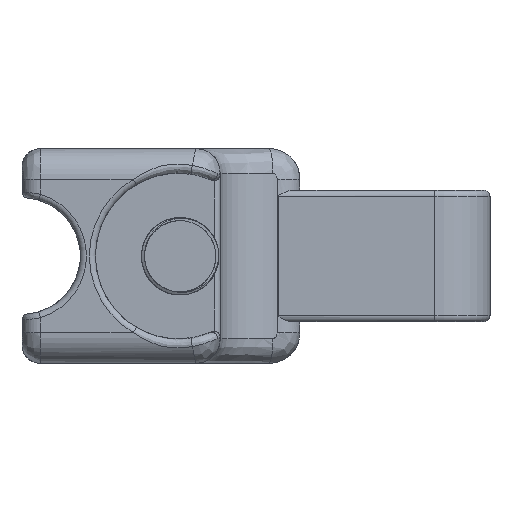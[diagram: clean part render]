
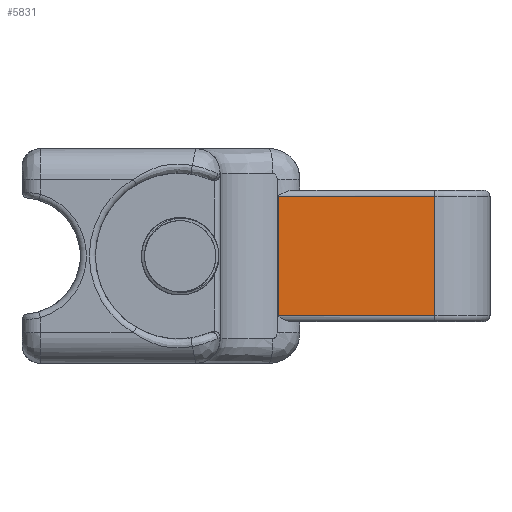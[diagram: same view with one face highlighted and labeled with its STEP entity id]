
A CAD part, left-side view. The second image highlights one B-rep face of the part: STEP entity #5831.
In plain terms, the highlighted planar face has unit normal (-1, 0, 0).
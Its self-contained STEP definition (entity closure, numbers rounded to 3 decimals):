
#237=PLANE('',#6344);
#534=FACE_OUTER_BOUND('',#863,.T.);
#863=EDGE_LOOP('',(#5238,#5239,#5240,#5241));
#1196=B_SPLINE_CURVE_WITH_KNOTS('',3,(#9870,#9871,#9872,#9873),
 .UNSPECIFIED.,.F.,.F.,(4,4),(0.05,1.995),
 .UNSPECIFIED.);
#1678=LINE('',#12551,#2162);
#1717=LINE('',#12905,#2201);
#1718=LINE('',#12908,#2202);
#2162=VECTOR('',#7611,10.);
#2201=VECTOR('',#7780,10.);
#2202=VECTOR('',#7785,10.);
#2416=VERTEX_POINT('',#9850);
#2417=VERTEX_POINT('',#9869);
#2708=VERTEX_POINT('',#12549);
#2759=VERTEX_POINT('',#12904);
#3045=EDGE_CURVE('',#2417,#2416,#1196,.T.);
#3514=EDGE_CURVE('',#2416,#2708,#1678,.T.);
#3600=EDGE_CURVE('',#2417,#2759,#1717,.T.);
#3602=EDGE_CURVE('',#2759,#2708,#1718,.T.);
#5238=ORIENTED_EDGE('',*,*,#3602,.F.);
#5239=ORIENTED_EDGE('',*,*,#3600,.F.);
#5240=ORIENTED_EDGE('',*,*,#3045,.T.);
#5241=ORIENTED_EDGE('',*,*,#3514,.T.);
#5831=ADVANCED_FACE('',(#534),#237,.F.);
#6344=AXIS2_PLACEMENT_3D('',#12907,#7783,#7784);
#7611=DIRECTION('',(0.,-1.,0.));
#7780=DIRECTION('',(0.,-1.,0.));
#7783=DIRECTION('center_axis',(1.,0.,0.));
#7784=DIRECTION('ref_axis',(0.,0.,-1.));
#7785=DIRECTION('',(0.,0.,-1.));
#9850=CARTESIAN_POINT('',(51.204,-20.772,7.775));
#9869=CARTESIAN_POINT('',(51.204,-20.772,27.225));
#9870=CARTESIAN_POINT('Ctrl Pts',(51.204,-20.772,27.225));
#9871=CARTESIAN_POINT('Ctrl Pts',(51.204,-20.772,20.742));
#9872=CARTESIAN_POINT('Ctrl Pts',(51.204,-20.772,14.258));
#9873=CARTESIAN_POINT('Ctrl Pts',(51.204,-20.772,7.775));
#12549=CARTESIAN_POINT('',(51.204,-46.239,7.775));
#12551=CARTESIAN_POINT('',(51.204,-24.239,7.775));
#12904=CARTESIAN_POINT('',(51.204,-46.239,27.225));
#12905=CARTESIAN_POINT('',(51.204,-24.239,27.225));
#12907=CARTESIAN_POINT('Origin',(51.204,-24.239,35.));
#12908=CARTESIAN_POINT('',(51.204,-46.239,26.25));
